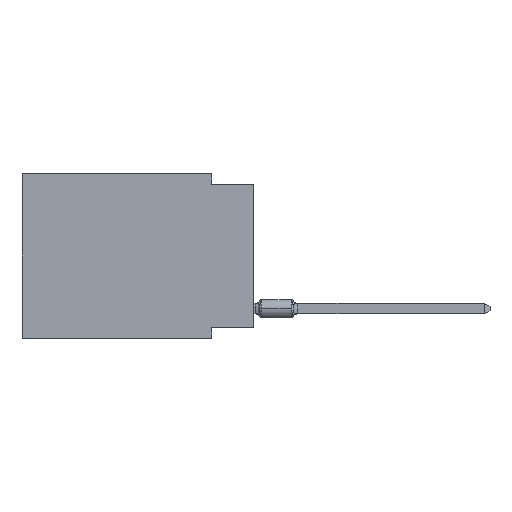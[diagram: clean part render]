
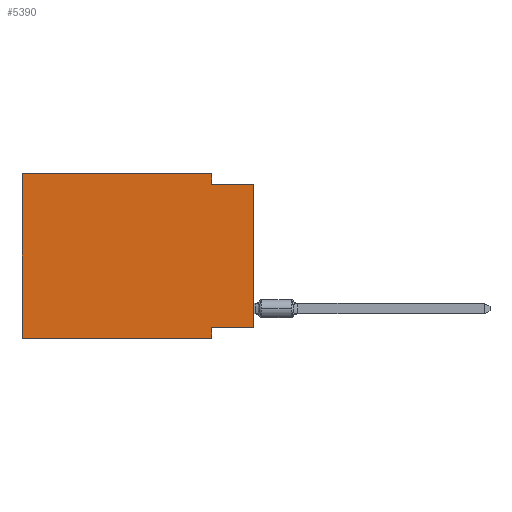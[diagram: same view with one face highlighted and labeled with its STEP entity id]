
A CAD part, left-side view. The second image highlights one B-rep face of the part: STEP entity #5390.
In plain terms, the highlighted planar face has unit normal (-1, 0, 0).
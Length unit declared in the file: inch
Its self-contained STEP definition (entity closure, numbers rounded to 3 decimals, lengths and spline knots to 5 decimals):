
#292 = CARTESIAN_POINT ( 'NONE',  ( 0., 0., -0.365 ) ) ;
#798 = VERTEX_POINT ( 'NONE', #10115 ) ;
#1280 = VERTEX_POINT ( 'NONE', #7203 ) ;
#1785 = LINE ( 'NONE', #8383, #2107 ) ;
#1965 = CARTESIAN_POINT ( 'NONE',  ( 0., 0.55, -0.39 ) ) ;
#2107 = VECTOR ( 'NONE', #16163, 39.37008 ) ;
#2925 = CARTESIAN_POINT ( 'NONE',  ( 0., 0.55, 0. ) ) ;
#3118 = LINE ( 'NONE', #10988, #16045 ) ;
#3403 = CARTESIAN_POINT ( 'NONE',  ( 0., 0.1, -0.025 ) ) ;
#3449 = VECTOR ( 'NONE', #15800, 39.37008 ) ;
#3594 = DIRECTION ( 'NONE',  ( 0., -1., 0. ) ) ;
#4083 = LINE ( 'NONE', #5132, #3449 ) ;
#4144 = DIRECTION ( 'NONE',  ( 0., 0., -1. ) ) ;
#4166 = VERTEX_POINT ( 'NONE', #292 ) ;
#4992 = CARTESIAN_POINT ( 'NONE',  ( 0., 0., -0.025 ) ) ;
#5088 = EDGE_CURVE ( 'NONE', #4166, #8141, #5554, .T. ) ;
#5132 = CARTESIAN_POINT ( 'NONE',  ( 0., 0.1, 0. ) ) ;
#5293 = VERTEX_POINT ( 'NONE', #13756 ) ;
#5390 = ADVANCED_FACE ( 'NONE', ( #15462 ), #14346, .F. ) ;
#5458 = CARTESIAN_POINT ( 'NONE',  ( 0., 0.1, -0.39 ) ) ;
#5554 = LINE ( 'NONE', #10942, #16167 ) ;
#5813 = DIRECTION ( 'NONE',  ( 0., 0., 1. ) ) ;
#6408 = ORIENTED_EDGE ( 'NONE', *, *, #10212, .F. ) ;
#6900 = ORIENTED_EDGE ( 'NONE', *, *, #12911, .F. ) ;
#7161 = VECTOR ( 'NONE', #7385, 39.37008 ) ;
#7203 = CARTESIAN_POINT ( 'NONE',  ( 0., 0.55, 0. ) ) ;
#7385 = DIRECTION ( 'NONE',  ( 0., -1., 0. ) ) ;
#7597 = VECTOR ( 'NONE', #3594, 39.37008 ) ;
#7700 = VECTOR ( 'NONE', #8144, 39.37008 ) ;
#8141 = VERTEX_POINT ( 'NONE', #13564 ) ;
#8144 = DIRECTION ( 'NONE',  ( 0., 0., 1. ) ) ;
#8383 = CARTESIAN_POINT ( 'NONE',  ( 0., 0., -0.365 ) ) ;
#8972 = CARTESIAN_POINT ( 'NONE',  ( 0., 0.55, 0. ) ) ;
#9266 = ORIENTED_EDGE ( 'NONE', *, *, #13544, .F. ) ;
#9904 = EDGE_CURVE ( 'NONE', #12194, #8141, #15159, .T. ) ;
#10115 = CARTESIAN_POINT ( 'NONE',  ( 0., 0.1, -0.365 ) ) ;
#10188 = LINE ( 'NONE', #12845, #7597 ) ;
#10212 = EDGE_CURVE ( 'NONE', #15590, #1280, #14633, .T. ) ;
#10556 = ORIENTED_EDGE ( 'NONE', *, *, #12983, .T. ) ;
#10588 = DIRECTION ( 'NONE',  ( 0., 0., -1. ) ) ;
#10748 = AXIS2_PLACEMENT_3D ( 'NONE', #8972, #14184, #10588 ) ;
#10920 = EDGE_LOOP ( 'NONE', ( #13186, #14214, #9266, #12683, #6408, #10556, #6900, #14639 ) ) ;
#10942 = CARTESIAN_POINT ( 'NONE',  ( 0., 0., 0. ) ) ;
#10988 = CARTESIAN_POINT ( 'NONE',  ( 0., 0.1, -0.39 ) ) ;
#11589 = CARTESIAN_POINT ( 'NONE',  ( 0., 0.55, 0. ) ) ;
#12194 = VERTEX_POINT ( 'NONE', #3403 ) ;
#12683 = ORIENTED_EDGE ( 'NONE', *, *, #16466, .F. ) ;
#12759 = VECTOR ( 'NONE', #14237, 39.37008 ) ;
#12845 = CARTESIAN_POINT ( 'NONE',  ( 0., 0.55, -0.39 ) ) ;
#12911 = EDGE_CURVE ( 'NONE', #798, #13631, #3118, .T. ) ;
#12983 = EDGE_CURVE ( 'NONE', #15590, #13631, #10188, .T. ) ;
#13186 = ORIENTED_EDGE ( 'NONE', *, *, #5088, .T. ) ;
#13227 = EDGE_CURVE ( 'NONE', #4166, #798, #1785, .T. ) ;
#13544 = EDGE_CURVE ( 'NONE', #5293, #12194, #4083, .T. ) ;
#13564 = CARTESIAN_POINT ( 'NONE',  ( 0., 0., -0.025 ) ) ;
#13631 = VERTEX_POINT ( 'NONE', #5458 ) ;
#13756 = CARTESIAN_POINT ( 'NONE',  ( 0., 0.1, 0. ) ) ;
#14184 = DIRECTION ( 'NONE',  ( 1., 0., 0. ) ) ;
#14214 = ORIENTED_EDGE ( 'NONE', *, *, #9904, .F. ) ;
#14237 = DIRECTION ( 'NONE',  ( 0., -1., 0. ) ) ;
#14346 = PLANE ( 'NONE',  #10748 ) ;
#14633 = LINE ( 'NONE', #2925, #7700 ) ;
#14639 = ORIENTED_EDGE ( 'NONE', *, *, #13227, .F. ) ;
#15159 = LINE ( 'NONE', #4992, #7161 ) ;
#15462 = FACE_OUTER_BOUND ( 'NONE', #10920, .T. ) ;
#15590 = VERTEX_POINT ( 'NONE', #1965 ) ;
#15800 = DIRECTION ( 'NONE',  ( 0., 0., -1. ) ) ;
#16045 = VECTOR ( 'NONE', #4144, 39.37008 ) ;
#16163 = DIRECTION ( 'NONE',  ( 0., 1., 0. ) ) ;
#16167 = VECTOR ( 'NONE', #5813, 39.37008 ) ;
#16466 = EDGE_CURVE ( 'NONE', #1280, #5293, #16804, .T. ) ;
#16804 = LINE ( 'NONE', #11589, #12759 ) ;
